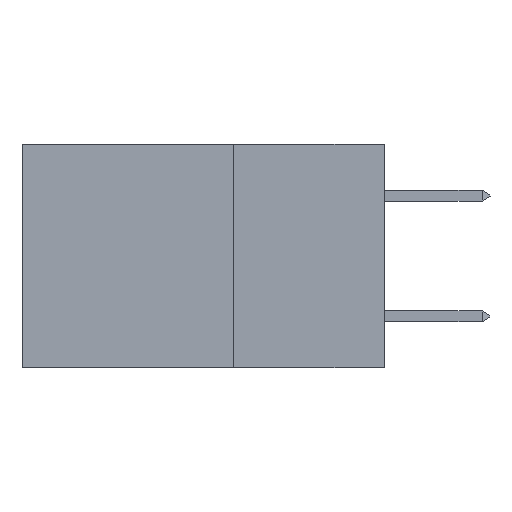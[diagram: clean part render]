
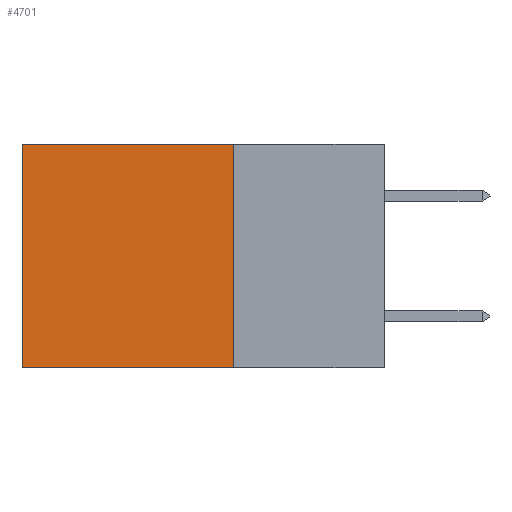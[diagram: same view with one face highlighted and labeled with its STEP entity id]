
A CAD part, left-side view. The second image highlights one B-rep face of the part: STEP entity #4701.
In plain terms, the highlighted planar face has unit normal (-1, 0, 0).
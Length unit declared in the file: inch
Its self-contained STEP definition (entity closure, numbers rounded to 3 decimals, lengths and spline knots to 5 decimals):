
#384 = LINE ( 'NONE', #26309, #11052 ) ;
#532 = VECTOR ( 'NONE', #34621, 39.37008 ) ;
#2075 = VERTEX_POINT ( 'NONE', #7668 ) ;
#3445 = LINE ( 'NONE', #32999, #14717 ) ;
#4701 = ADVANCED_FACE ( 'NONE', ( #21623 ), #31464, .F. ) ;
#5720 = DIRECTION ( 'NONE',  ( 0., 0., -1. ) ) ;
#7668 = CARTESIAN_POINT ( 'NONE',  ( 0.2875, 0.6, -0.37 ) ) ;
#8371 = DIRECTION ( 'NONE',  ( 1., 0., 0. ) ) ;
#9323 = DIRECTION ( 'NONE',  ( 0., 1., 0. ) ) ;
#10371 = LINE ( 'NONE', #21927, #14993 ) ;
#11052 = VECTOR ( 'NONE', #17600, 39.37008 ) ;
#14717 = VECTOR ( 'NONE', #9323, 39.37008 ) ;
#14993 = VECTOR ( 'NONE', #32743, 39.37008 ) ;
#16757 = ORIENTED_EDGE ( 'NONE', *, *, #17635, .F. ) ;
#16947 = VERTEX_POINT ( 'NONE', #23881 ) ;
#17600 = DIRECTION ( 'NONE',  ( 0., 1., 0. ) ) ;
#17635 = EDGE_CURVE ( 'NONE', #36975, #29820, #10371, .T. ) ;
#17960 = EDGE_CURVE ( 'NONE', #16947, #2075, #26440, .T. ) ;
#19904 = ORIENTED_EDGE ( 'NONE', *, *, #17960, .T. ) ;
#20818 = EDGE_LOOP ( 'NONE', ( #19904, #36418, #16757, #23996 ) ) ;
#21623 = FACE_OUTER_BOUND ( 'NONE', #20818, .T. ) ;
#21927 = CARTESIAN_POINT ( 'NONE',  ( 0.2875, 0.25, 0. ) ) ;
#22937 = CARTESIAN_POINT ( 'NONE',  ( 0.2875, 0.25, 0. ) ) ;
#23881 = CARTESIAN_POINT ( 'NONE',  ( 0.2875, 0.6, 0. ) ) ;
#23996 = ORIENTED_EDGE ( 'NONE', *, *, #24512, .T. ) ;
#24512 = EDGE_CURVE ( 'NONE', #36975, #16947, #384, .T. ) ;
#25949 = CARTESIAN_POINT ( 'NONE',  ( 0.2875, 0.25, 0. ) ) ;
#26309 = CARTESIAN_POINT ( 'NONE',  ( 0.2875, 0.25, 0. ) ) ;
#26440 = LINE ( 'NONE', #28918, #532 ) ;
#27450 = EDGE_CURVE ( 'NONE', #29820, #2075, #3445, .T. ) ;
#28918 = CARTESIAN_POINT ( 'NONE',  ( 0.2875, 0.6, 0. ) ) ;
#29820 = VERTEX_POINT ( 'NONE', #30077 ) ;
#30077 = CARTESIAN_POINT ( 'NONE',  ( 0.2875, 0.25, -0.37 ) ) ;
#31464 = PLANE ( 'NONE',  #32427 ) ;
#32427 = AXIS2_PLACEMENT_3D ( 'NONE', #22937, #8371, #5720 ) ;
#32743 = DIRECTION ( 'NONE',  ( 0., 0., -1. ) ) ;
#32999 = CARTESIAN_POINT ( 'NONE',  ( 0.2875, 0.25, -0.37 ) ) ;
#34621 = DIRECTION ( 'NONE',  ( 0., 0., -1. ) ) ;
#36418 = ORIENTED_EDGE ( 'NONE', *, *, #27450, .F. ) ;
#36975 = VERTEX_POINT ( 'NONE', #25949 ) ;
